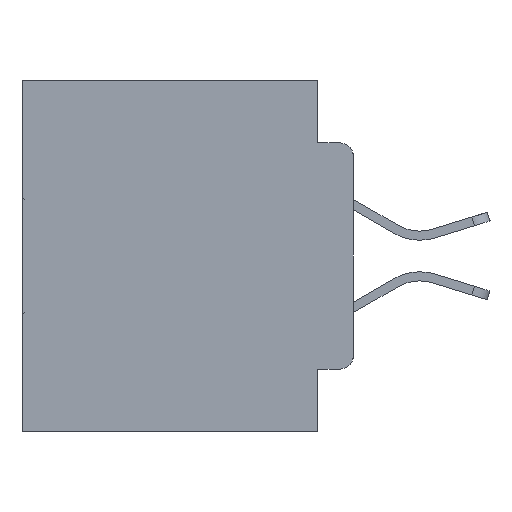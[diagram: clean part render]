
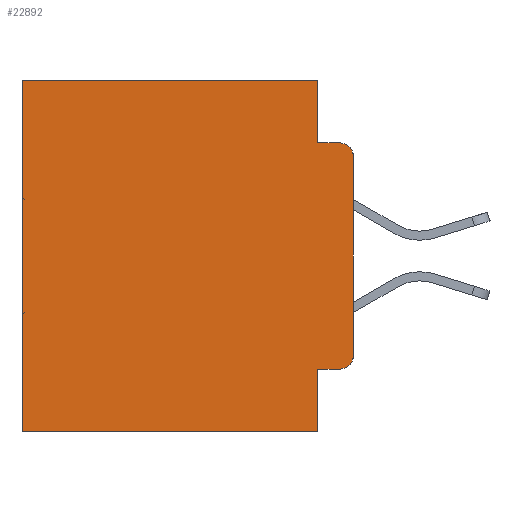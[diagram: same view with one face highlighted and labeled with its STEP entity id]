
A CAD part, left-side view. The second image highlights one B-rep face of the part: STEP entity #22892.
In plain terms, the highlighted planar face has unit normal (-1, 0, 0).
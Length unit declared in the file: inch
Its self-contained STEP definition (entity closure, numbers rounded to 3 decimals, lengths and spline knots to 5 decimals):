
#398 = CARTESIAN_POINT ( 'NONE',  ( 0.298, 0., 0. ) ) ;
#640 = EDGE_CURVE ( 'NONE', #8044, #2742, #11399, .T. ) ;
#1009 = CARTESIAN_POINT ( 'NONE',  ( 0.298, 0., -0.5 ) ) ;
#1414 = EDGE_CURVE ( 'NONE', #25857, #3486, #8663, .T. ) ;
#2460 = VECTOR ( 'NONE', #7207, 39.37008 ) ;
#2541 = ORIENTED_EDGE ( 'NONE', *, *, #20584, .T. ) ;
#2742 = VERTEX_POINT ( 'NONE', #5798 ) ;
#3370 = VECTOR ( 'NONE', #17957, 39.37008 ) ;
#3486 = VERTEX_POINT ( 'NONE', #25861 ) ;
#3676 = CARTESIAN_POINT ( 'NONE',  ( 0.298, 0.02, -0.1085 ) ) ;
#4150 = EDGE_CURVE ( 'NONE', #16667, #22124, #10747, .T. ) ;
#4346 = CARTESIAN_POINT ( 'NONE',  ( 0.298, 0.051, -0.0885 ) ) ;
#4763 = CIRCLE ( 'NONE', #21220, 0.02 ) ;
#4986 = CARTESIAN_POINT ( 'NONE',  ( 0.298, 0.473, 0. ) ) ;
#5239 = LINE ( 'NONE', #24411, #17517 ) ;
#5299 = CARTESIAN_POINT ( 'NONE',  ( 0.298, 0.051, -0.5 ) ) ;
#5396 = AXIS2_PLACEMENT_3D ( 'NONE', #3676, #20782, #6184 ) ;
#5798 = CARTESIAN_POINT ( 'NONE',  ( 0.298, 0.02, -0.0885 ) ) ;
#6184 = DIRECTION ( 'NONE',  ( 0., 0., -1. ) ) ;
#6835 = ORIENTED_EDGE ( 'NONE', *, *, #640, .F. ) ;
#7207 = DIRECTION ( 'NONE',  ( 0., 0., -1. ) ) ;
#8044 = VERTEX_POINT ( 'NONE', #25035 ) ;
#8428 = VECTOR ( 'NONE', #19001, 39.37008 ) ;
#8510 = VECTOR ( 'NONE', #18181, 39.37008 ) ;
#8663 = LINE ( 'NONE', #27280, #15930 ) ;
#9249 = ORIENTED_EDGE ( 'NONE', *, *, #16023, .F. ) ;
#9820 = CIRCLE ( 'NONE', #5396, 0.02 ) ;
#9961 = ORIENTED_EDGE ( 'NONE', *, *, #30620, .T. ) ;
#10299 = VERTEX_POINT ( 'NONE', #4986 ) ;
#10621 = VECTOR ( 'NONE', #14277, 39.37008 ) ;
#10747 = LINE ( 'NONE', #13262, #3370 ) ;
#11034 = VECTOR ( 'NONE', #18221, 39.37008 ) ;
#11123 = DIRECTION ( 'NONE',  ( -1., 0., 0. ) ) ;
#11251 = CARTESIAN_POINT ( 'NONE',  ( 0.298, 0., -0.1085 ) ) ;
#11399 = LINE ( 'NONE', #4346, #10621 ) ;
#11732 = EDGE_CURVE ( 'NONE', #23440, #10299, #15013, .T. ) ;
#12163 = CARTESIAN_POINT ( 'NONE',  ( 0.298, 0.02, -0.4115 ) ) ;
#12866 = DIRECTION ( 'NONE',  ( 0., 0., -1. ) ) ;
#13262 = CARTESIAN_POINT ( 'NONE',  ( 0.298, 0.051, -0.4115 ) ) ;
#14123 = EDGE_CURVE ( 'NONE', #23440, #8044, #5239, .T. ) ;
#14277 = DIRECTION ( 'NONE',  ( 0., -1., 0. ) ) ;
#14905 = ORIENTED_EDGE ( 'NONE', *, *, #11732, .T. ) ;
#15013 = LINE ( 'NONE', #15770, #8510 ) ;
#15079 = ORIENTED_EDGE ( 'NONE', *, *, #1414, .F. ) ;
#15602 = LINE ( 'NONE', #21684, #2460 ) ;
#15770 = CARTESIAN_POINT ( 'NONE',  ( 0.298, 0., 0. ) ) ;
#15930 = VECTOR ( 'NONE', #27526, 39.37008 ) ;
#16023 = EDGE_CURVE ( 'NONE', #20890, #23200, #17515, .T. ) ;
#16298 = EDGE_CURVE ( 'NONE', #16667, #20890, #15602, .T. ) ;
#16583 = CARTESIAN_POINT ( 'NONE',  ( 0.298, 0.473, 0. ) ) ;
#16667 = VERTEX_POINT ( 'NONE', #27743 ) ;
#17234 = EDGE_CURVE ( 'NONE', #25857, #2742, #9820, .T. ) ;
#17278 = ORIENTED_EDGE ( 'NONE', *, *, #4150, .T. ) ;
#17515 = LINE ( 'NONE', #1009, #11034 ) ;
#17517 = VECTOR ( 'NONE', #26752, 39.37008 ) ;
#17957 = DIRECTION ( 'NONE',  ( 0., -1., 0. ) ) ;
#18181 = DIRECTION ( 'NONE',  ( 0., 1., 0. ) ) ;
#18221 = DIRECTION ( 'NONE',  ( 0., 1., 0. ) ) ;
#19001 = DIRECTION ( 'NONE',  ( 0., 0., -1. ) ) ;
#20584 = EDGE_CURVE ( 'NONE', #10299, #23200, #21346, .T. ) ;
#20728 = ORIENTED_EDGE ( 'NONE', *, *, #17234, .T. ) ;
#20782 = DIRECTION ( 'NONE',  ( -1., 0., 0. ) ) ;
#20890 = VERTEX_POINT ( 'NONE', #5299 ) ;
#21220 = AXIS2_PLACEMENT_3D ( 'NONE', #25540, #11123, #27893 ) ;
#21274 = AXIS2_PLACEMENT_3D ( 'NONE', #398, #27197, #12866 ) ;
#21346 = LINE ( 'NONE', #16583, #8428 ) ;
#21684 = CARTESIAN_POINT ( 'NONE',  ( 0.298, 0.051, 0. ) ) ;
#22124 = VERTEX_POINT ( 'NONE', #12163 ) ;
#22892 = ADVANCED_FACE ( 'NONE', ( #23852 ), #24848, .F. ) ;
#23200 = VERTEX_POINT ( 'NONE', #28315 ) ;
#23440 = VERTEX_POINT ( 'NONE', #24922 ) ;
#23852 = FACE_OUTER_BOUND ( 'NONE', #28941, .T. ) ;
#24411 = CARTESIAN_POINT ( 'NONE',  ( 0.298, 0.051, 0. ) ) ;
#24848 = PLANE ( 'NONE',  #21274 ) ;
#24922 = CARTESIAN_POINT ( 'NONE',  ( 0.298, 0.051, 0. ) ) ;
#25035 = CARTESIAN_POINT ( 'NONE',  ( 0.298, 0.051, -0.0885 ) ) ;
#25540 = CARTESIAN_POINT ( 'NONE',  ( 0.298, 0.02, -0.3915 ) ) ;
#25857 = VERTEX_POINT ( 'NONE', #11251 ) ;
#25861 = CARTESIAN_POINT ( 'NONE',  ( 0.298, 0., -0.3915 ) ) ;
#26752 = DIRECTION ( 'NONE',  ( 0., 0., -1. ) ) ;
#27197 = DIRECTION ( 'NONE',  ( 1., 0., 0. ) ) ;
#27280 = CARTESIAN_POINT ( 'NONE',  ( 0.298, 0., 0. ) ) ;
#27526 = DIRECTION ( 'NONE',  ( 0., 0., -1. ) ) ;
#27675 = ORIENTED_EDGE ( 'NONE', *, *, #14123, .F. ) ;
#27743 = CARTESIAN_POINT ( 'NONE',  ( 0.298, 0.051, -0.4115 ) ) ;
#27893 = DIRECTION ( 'NONE',  ( 0., 0., -1. ) ) ;
#28315 = CARTESIAN_POINT ( 'NONE',  ( 0.298, 0.473, -0.5 ) ) ;
#28339 = ORIENTED_EDGE ( 'NONE', *, *, #16298, .F. ) ;
#28941 = EDGE_LOOP ( 'NONE', ( #15079, #20728, #6835, #27675, #14905, #2541, #9249, #28339, #17278, #9961 ) ) ;
#30620 = EDGE_CURVE ( 'NONE', #22124, #3486, #4763, .T. ) ;
